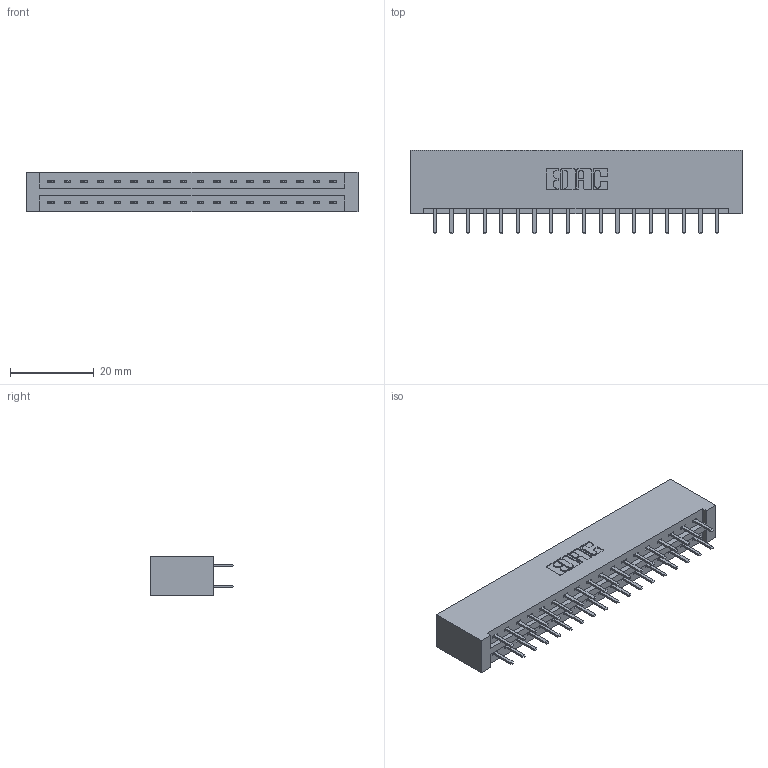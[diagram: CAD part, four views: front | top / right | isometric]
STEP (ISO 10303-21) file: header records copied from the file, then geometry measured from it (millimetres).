
FILE_DESCRIPTION (( 'STEP AP203' ), '1' );
FILE_NAME ('387-036-520-201.STEP', '2019-10-17T18:36:06', ( '' ), ( '' ), 'SwSTEP 2.0', 'SolidWorks 2016', '' );
FILE_SCHEMA (( 'CONFIG_CONTROL_DESIGN' ));
Length unit declared in the file: inch
Products named in the file (3): 337 Part_No Mounting Lugs; 387-036-520-201; 345-292-001_345-293-120
Assembly tree (37 placements, depth 2):
  387-036-520-201
    337 Part_No Mounting Lugs
    345-292-001_345-293-120  x36
Bounding box: 79.2 x 20.02 x 9.4 mm (x, y, z)
Volume: 8771.9 mm3; surface area: 9694.5 mm2
Topology: 37 solids, 37 shells, 2194 faces, 6371 edges, 4150 vertices
Faces by surface type: plane 1506, cylinder 688
Entity records: 16897 total; most frequent: CARTESIAN_POINT 2878, ORIENTED_EDGE 2802, DIRECTION 2473, EDGE_CURVE 1401, LINE 1277, VECTOR 1277, VERTEX_POINT 930, AXIS2_PLACEMENT_3D 598
